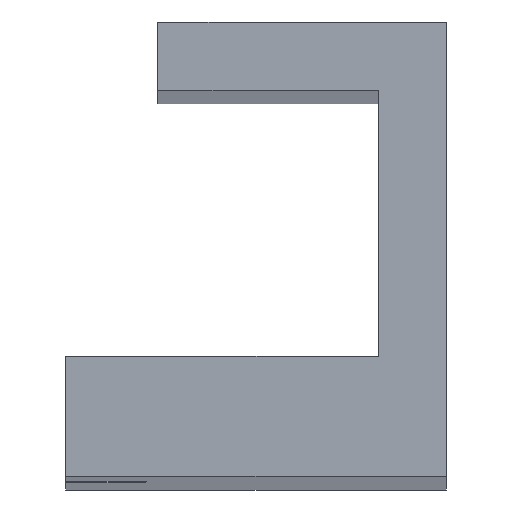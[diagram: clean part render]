
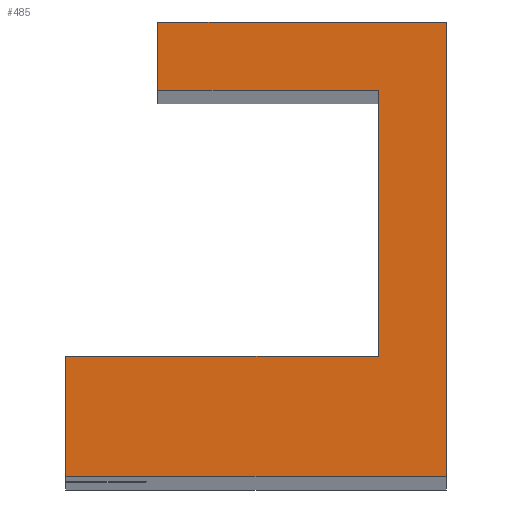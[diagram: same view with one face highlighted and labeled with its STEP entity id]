
A CAD part, top view. The second image highlights one B-rep face of the part: STEP entity #485.
In plain terms, the highlighted planar face has unit normal (0, 0, 1).
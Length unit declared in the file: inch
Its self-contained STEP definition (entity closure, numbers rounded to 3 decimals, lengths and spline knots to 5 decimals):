
#71=FACE_OUTER_BOUND('',#93,.T.);
#93=EDGE_LOOP('',(#371,#372,#373,#374,#375,#376,#377,#378));
#126=LINE('',#712,#170);
#139=LINE('',#739,#183);
#147=LINE('',#754,#191);
#150=LINE('',#761,#194);
#151=LINE('',#763,#195);
#152=LINE('',#765,#196);
#153=LINE('',#767,#197);
#154=LINE('',#768,#198);
#170=VECTOR('',#572,0.3937);
#183=VECTOR('',#591,0.3937);
#191=VECTOR('',#603,0.3937);
#194=VECTOR('',#612,0.3937);
#195=VECTOR('',#613,0.3937);
#196=VECTOR('',#614,0.3937);
#197=VECTOR('',#615,0.3937);
#198=VECTOR('',#616,0.3937);
#212=VERTEX_POINT('',#706);
#214=VERTEX_POINT('',#710);
#225=VERTEX_POINT('',#737);
#230=VERTEX_POINT('',#753);
#231=VERTEX_POINT('',#760);
#232=VERTEX_POINT('',#762);
#233=VERTEX_POINT('',#764);
#234=VERTEX_POINT('',#766);
#262=EDGE_CURVE('',#212,#214,#126,.T.);
#275=EDGE_CURVE('',#225,#214,#139,.T.);
#283=EDGE_CURVE('',#212,#230,#147,.T.);
#286=EDGE_CURVE('',#231,#225,#150,.T.);
#287=EDGE_CURVE('',#232,#231,#151,.T.);
#288=EDGE_CURVE('',#233,#232,#152,.T.);
#289=EDGE_CURVE('',#234,#233,#153,.T.);
#290=EDGE_CURVE('',#230,#234,#154,.T.);
#371=ORIENTED_EDGE('',*,*,#262,.T.);
#372=ORIENTED_EDGE('',*,*,#275,.F.);
#373=ORIENTED_EDGE('',*,*,#286,.F.);
#374=ORIENTED_EDGE('',*,*,#287,.F.);
#375=ORIENTED_EDGE('',*,*,#288,.F.);
#376=ORIENTED_EDGE('',*,*,#289,.F.);
#377=ORIENTED_EDGE('',*,*,#290,.F.);
#378=ORIENTED_EDGE('',*,*,#283,.F.);
#471=PLANE('',#527);
#485=ADVANCED_FACE('',(#71),#471,.F.);
#527=AXIS2_PLACEMENT_3D('',#759,#610,#611);
#572=DIRECTION('',(0.,-1.,0.));
#591=DIRECTION('',(-1.,0.,0.));
#603=DIRECTION('',(1.,0.,0.));
#610=DIRECTION('center_axis',(0.,0.,-1.));
#611=DIRECTION('ref_axis',(-1.,0.,0.));
#612=DIRECTION('',(0.,-1.,0.));
#613=DIRECTION('',(1.,0.,0.));
#614=DIRECTION('',(0.,1.,0.));
#615=DIRECTION('',(-1.,0.,0.));
#616=DIRECTION('',(0.,1.,0.));
#706=CARTESIAN_POINT('',(0.05,0.10406,6.80194));
#710=CARTESIAN_POINT('',(0.05,0.,6.80194));
#712=CARTESIAN_POINT('',(0.05,0.1305,6.80194));
#737=CARTESIAN_POINT('',(0.38,0.,6.80194));
#739=CARTESIAN_POINT('',(0.095,0.,6.80194));
#753=CARTESIAN_POINT('',(0.32094,0.10406,6.80194));
#754=CARTESIAN_POINT('',(0.,0.10406,6.80194));
#759=CARTESIAN_POINT('Origin',(0.19,0.19685,6.80194));
#760=CARTESIAN_POINT('',(0.38,0.3937,6.80194));
#761=CARTESIAN_POINT('',(0.38,0.09843,6.80194));
#762=CARTESIAN_POINT('',(0.13,0.3937,6.80194));
#763=CARTESIAN_POINT('',(0.285,0.3937,6.80194));
#764=CARTESIAN_POINT('',(0.13,0.33465,6.80194));
#765=CARTESIAN_POINT('',(0.13,0.26575,6.80194));
#766=CARTESIAN_POINT('',(0.32094,0.33465,6.80194));
#767=CARTESIAN_POINT('',(0.145,0.33465,6.80194));
#768=CARTESIAN_POINT('',(0.32094,0.26575,6.80194));
